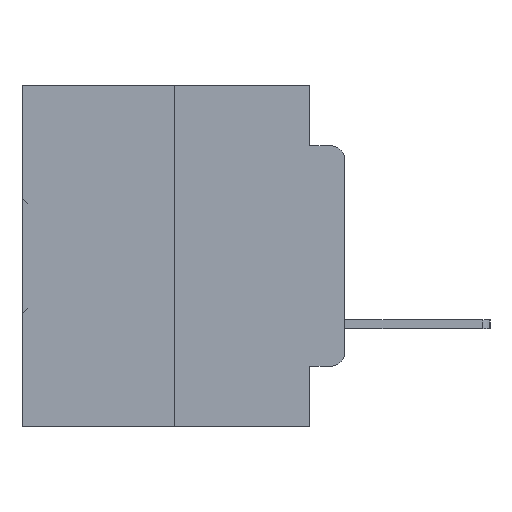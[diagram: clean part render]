
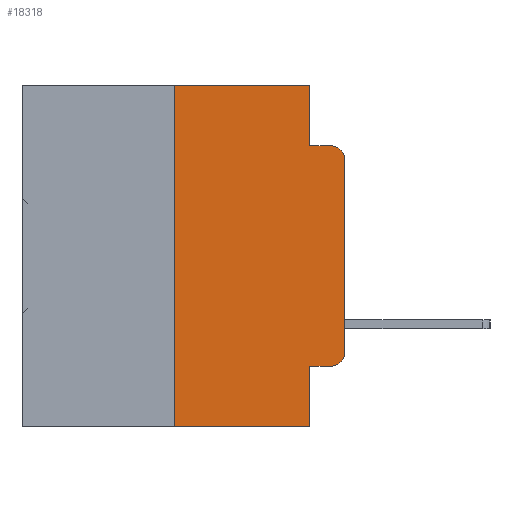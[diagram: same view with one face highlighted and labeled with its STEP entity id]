
A CAD part, left-side view. The second image highlights one B-rep face of the part: STEP entity #18318.
In plain terms, the highlighted planar face has unit normal (-1, 0, 0).
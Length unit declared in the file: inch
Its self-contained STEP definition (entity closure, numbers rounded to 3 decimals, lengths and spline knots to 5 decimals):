
#354 = DIRECTION ( 'NONE',  ( 0., -1., 0. ) ) ;
#636 = CARTESIAN_POINT ( 'NONE',  ( 0., 0.051, 0. ) ) ;
#1119 = CARTESIAN_POINT ( 'NONE',  ( 0., 0.473, 0. ) ) ;
#1472 = DIRECTION ( 'NONE',  ( 0., 0., -1. ) ) ;
#1547 = LINE ( 'NONE', #5229, #9682 ) ;
#2427 = VERTEX_POINT ( 'NONE', #20650 ) ;
#2936 = DIRECTION ( 'NONE',  ( 0., 0., -1. ) ) ;
#3096 = LINE ( 'NONE', #26706, #30451 ) ;
#3431 = EDGE_CURVE ( 'NONE', #17096, #20549, #11620, .T. ) ;
#3871 = DIRECTION ( 'NONE',  ( 0., 0., -1. ) ) ;
#5229 = CARTESIAN_POINT ( 'NONE',  ( 0., 0.25, 0. ) ) ;
#5233 = VECTOR ( 'NONE', #5950, 39.37008 ) ;
#5283 = EDGE_CURVE ( 'NONE', #12445, #17096, #32024, .T. ) ;
#5746 = CARTESIAN_POINT ( 'NONE',  ( 0., 0.473, -0.5 ) ) ;
#5950 = DIRECTION ( 'NONE',  ( 0., 0., -1. ) ) ;
#5977 = AXIS2_PLACEMENT_3D ( 'NONE', #1119, #19858, #3871 ) ;
#5987 = CARTESIAN_POINT ( 'NONE',  ( 0., 0., -0.1085 ) ) ;
#6489 = VERTEX_POINT ( 'NONE', #636 ) ;
#7701 = DIRECTION ( 'NONE',  ( 0., 0., 1. ) ) ;
#8232 = CARTESIAN_POINT ( 'NONE',  ( 0., 0., 0. ) ) ;
#8454 = ORIENTED_EDGE ( 'NONE', *, *, #34143, .F. ) ;
#8774 = VECTOR ( 'NONE', #16414, 39.37008 ) ;
#9514 = VECTOR ( 'NONE', #354, 39.37008 ) ;
#9682 = VECTOR ( 'NONE', #21150, 39.37008 ) ;
#9704 = ORIENTED_EDGE ( 'NONE', *, *, #3431, .T. ) ;
#10278 = ORIENTED_EDGE ( 'NONE', *, *, #23729, .F. ) ;
#10453 = VERTEX_POINT ( 'NONE', #26552 ) ;
#10556 = LINE ( 'NONE', #15802, #31450 ) ;
#10659 = DIRECTION ( 'NONE',  ( 0., -1., 0. ) ) ;
#10959 = DIRECTION ( 'NONE',  ( 0., -1., 0. ) ) ;
#11289 = VERTEX_POINT ( 'NONE', #14758 ) ;
#11620 = CIRCLE ( 'NONE', #11970, 0.02 ) ;
#11708 = CARTESIAN_POINT ( 'NONE',  ( 0., 0., -0.3915 ) ) ;
#11933 = PLANE ( 'NONE',  #5977 ) ;
#11970 = AXIS2_PLACEMENT_3D ( 'NONE', #31962, #31916, #1472 ) ;
#12270 = DIRECTION ( 'NONE',  ( -1., 0., 0. ) ) ;
#12445 = VERTEX_POINT ( 'NONE', #11708 ) ;
#13188 = AXIS2_PLACEMENT_3D ( 'NONE', #28022, #12270, #30610 ) ;
#13293 = VECTOR ( 'NONE', #2936, 39.37008 ) ;
#13368 = LINE ( 'NONE', #27000, #8774 ) ;
#13865 = CARTESIAN_POINT ( 'NONE',  ( 0., 0.02, -0.0885 ) ) ;
#14758 = CARTESIAN_POINT ( 'NONE',  ( 0., 0.051, -0.0885 ) ) ;
#14971 = VERTEX_POINT ( 'NONE', #17423 ) ;
#15802 = CARTESIAN_POINT ( 'NONE',  ( 0., 0.473, 0. ) ) ;
#16414 = DIRECTION ( 'NONE',  ( 0., -1., 0. ) ) ;
#16502 = LINE ( 'NONE', #5746, #9514 ) ;
#17096 = VERTEX_POINT ( 'NONE', #5987 ) ;
#17119 = CIRCLE ( 'NONE', #13188, 0.02 ) ;
#17398 = ORIENTED_EDGE ( 'NONE', *, *, #18401, .T. ) ;
#17423 = CARTESIAN_POINT ( 'NONE',  ( 0., 0.25, 0. ) ) ;
#17446 = ORIENTED_EDGE ( 'NONE', *, *, #21973, .T. ) ;
#18318 = ADVANCED_FACE ( 'NONE', ( #18758 ), #11933, .F. ) ;
#18380 = ORIENTED_EDGE ( 'NONE', *, *, #5283, .T. ) ;
#18401 = EDGE_CURVE ( 'NONE', #27039, #12445, #17119, .T. ) ;
#18662 = EDGE_CURVE ( 'NONE', #14971, #6489, #10556, .T. ) ;
#18758 = FACE_OUTER_BOUND ( 'NONE', #25015, .T. ) ;
#18917 = VECTOR ( 'NONE', #7701, 39.37008 ) ;
#19516 = CARTESIAN_POINT ( 'NONE',  ( 0., 0.051, -0.5 ) ) ;
#19535 = ORIENTED_EDGE ( 'NONE', *, *, #25500, .F. ) ;
#19858 = DIRECTION ( 'NONE',  ( 1., 0., 0. ) ) ;
#19974 = ORIENTED_EDGE ( 'NONE', *, *, #18662, .F. ) ;
#20108 = CARTESIAN_POINT ( 'NONE',  ( 0., 0.02, -0.4115 ) ) ;
#20549 = VERTEX_POINT ( 'NONE', #13865 ) ;
#20650 = CARTESIAN_POINT ( 'NONE',  ( 0., 0.051, -0.4115 ) ) ;
#21150 = DIRECTION ( 'NONE',  ( 0., 0., 1. ) ) ;
#21860 = CARTESIAN_POINT ( 'NONE',  ( 0., 0.051, 0. ) ) ;
#21973 = EDGE_CURVE ( 'NONE', #2427, #27039, #13368, .T. ) ;
#22087 = ORIENTED_EDGE ( 'NONE', *, *, #27252, .F. ) ;
#23729 = EDGE_CURVE ( 'NONE', #2427, #23820, #32439, .T. ) ;
#23820 = VERTEX_POINT ( 'NONE', #19516 ) ;
#25015 = EDGE_LOOP ( 'NONE', ( #18380, #9704, #8454, #22087, #19974, #19535, #29599, #10278, #17446, #17398 ) ) ;
#25500 = EDGE_CURVE ( 'NONE', #10453, #14971, #1547, .T. ) ;
#26552 = CARTESIAN_POINT ( 'NONE',  ( 0., 0.25, -0.5 ) ) ;
#26706 = CARTESIAN_POINT ( 'NONE',  ( 0., 0.051, -0.0885 ) ) ;
#27000 = CARTESIAN_POINT ( 'NONE',  ( 0., 0.051, -0.4115 ) ) ;
#27039 = VERTEX_POINT ( 'NONE', #20108 ) ;
#27249 = LINE ( 'NONE', #31975, #13293 ) ;
#27252 = EDGE_CURVE ( 'NONE', #6489, #11289, #27249, .T. ) ;
#28022 = CARTESIAN_POINT ( 'NONE',  ( 0., 0.02, -0.3915 ) ) ;
#29599 = ORIENTED_EDGE ( 'NONE', *, *, #31177, .T. ) ;
#30451 = VECTOR ( 'NONE', #10959, 39.37008 ) ;
#30610 = DIRECTION ( 'NONE',  ( 0., 0., -1. ) ) ;
#31177 = EDGE_CURVE ( 'NONE', #10453, #23820, #16502, .T. ) ;
#31450 = VECTOR ( 'NONE', #10659, 39.37008 ) ;
#31916 = DIRECTION ( 'NONE',  ( -1., 0., 0. ) ) ;
#31962 = CARTESIAN_POINT ( 'NONE',  ( 0., 0.02, -0.1085 ) ) ;
#31975 = CARTESIAN_POINT ( 'NONE',  ( 0., 0.051, 0. ) ) ;
#32024 = LINE ( 'NONE', #8232, #18917 ) ;
#32439 = LINE ( 'NONE', #21860, #5233 ) ;
#34143 = EDGE_CURVE ( 'NONE', #11289, #20549, #3096, .T. ) ;
